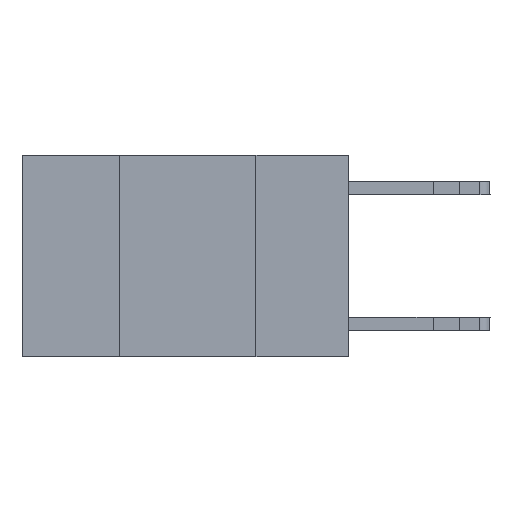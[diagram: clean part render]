
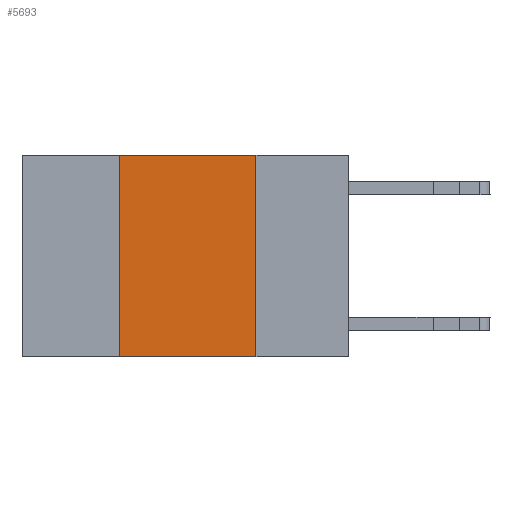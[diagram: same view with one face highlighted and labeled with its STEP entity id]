
A CAD part, left-side view. The second image highlights one B-rep face of the part: STEP entity #5693.
In plain terms, the highlighted planar face has unit normal (-1, 0, 0).
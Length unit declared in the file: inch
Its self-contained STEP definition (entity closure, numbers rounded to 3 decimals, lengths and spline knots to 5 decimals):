
#1095 = DIRECTION ( 'NONE',  ( 0., 0., -1. ) ) ;
#2667 = VERTEX_POINT ( 'NONE', #22265 ) ;
#3144 = DIRECTION ( 'NONE',  ( 0., 0., -1. ) ) ;
#3331 = ORIENTED_EDGE ( 'NONE', *, *, #19190, .T. ) ;
#4666 = CARTESIAN_POINT ( 'NONE',  ( 0., 0.42, 0. ) ) ;
#4745 = LINE ( 'NONE', #8666, #14378 ) ;
#5693 = ADVANCED_FACE ( 'NONE', ( #14031 ), #21693, .F. ) ;
#7227 = VERTEX_POINT ( 'NONE', #11358 ) ;
#8262 = EDGE_CURVE ( 'NONE', #22435, #7227, #21835, .T. ) ;
#8624 = ORIENTED_EDGE ( 'NONE', *, *, #17405, .F. ) ;
#8666 = CARTESIAN_POINT ( 'NONE',  ( 0., 0.17, 0. ) ) ;
#8947 = CARTESIAN_POINT ( 'NONE',  ( 0., 0.6, -0.37 ) ) ;
#10653 = LINE ( 'NONE', #8947, #11462 ) ;
#10906 = DIRECTION ( 'NONE',  ( 0., -1., 0. ) ) ;
#11358 = CARTESIAN_POINT ( 'NONE',  ( 0., 0.17, 0. ) ) ;
#11462 = VECTOR ( 'NONE', #18292, 39.37008 ) ;
#14021 = EDGE_CURVE ( 'NONE', #7227, #21128, #4745, .T. ) ;
#14031 = FACE_OUTER_BOUND ( 'NONE', #23210, .T. ) ;
#14378 = VECTOR ( 'NONE', #3144, 39.37008 ) ;
#14428 = CARTESIAN_POINT ( 'NONE',  ( 0., 0.6, 0. ) ) ;
#15342 = AXIS2_PLACEMENT_3D ( 'NONE', #21444, #17814, #1095 ) ;
#16027 = DIRECTION ( 'NONE',  ( 0., 0., 1. ) ) ;
#16796 = VECTOR ( 'NONE', #10906, 39.37008 ) ;
#16872 = VECTOR ( 'NONE', #16027, 39.37008 ) ;
#17222 = ORIENTED_EDGE ( 'NONE', *, *, #14021, .F. ) ;
#17405 = EDGE_CURVE ( 'NONE', #2667, #22435, #19899, .T. ) ;
#17814 = DIRECTION ( 'NONE',  ( 1., 0., 0. ) ) ;
#17952 = CARTESIAN_POINT ( 'NONE',  ( 0., 0.42, 0. ) ) ;
#18292 = DIRECTION ( 'NONE',  ( 0., -1., 0. ) ) ;
#19190 = EDGE_CURVE ( 'NONE', #2667, #21128, #10653, .T. ) ;
#19899 = LINE ( 'NONE', #17952, #16872 ) ;
#20258 = ORIENTED_EDGE ( 'NONE', *, *, #8262, .F. ) ;
#20479 = CARTESIAN_POINT ( 'NONE',  ( 0., 0.17, -0.37 ) ) ;
#21128 = VERTEX_POINT ( 'NONE', #20479 ) ;
#21444 = CARTESIAN_POINT ( 'NONE',  ( 0., 0.6, 0. ) ) ;
#21693 = PLANE ( 'NONE',  #15342 ) ;
#21835 = LINE ( 'NONE', #14428, #16796 ) ;
#22265 = CARTESIAN_POINT ( 'NONE',  ( 0., 0.42, -0.37 ) ) ;
#22435 = VERTEX_POINT ( 'NONE', #4666 ) ;
#23210 = EDGE_LOOP ( 'NONE', ( #17222, #20258, #8624, #3331 ) ) ;
